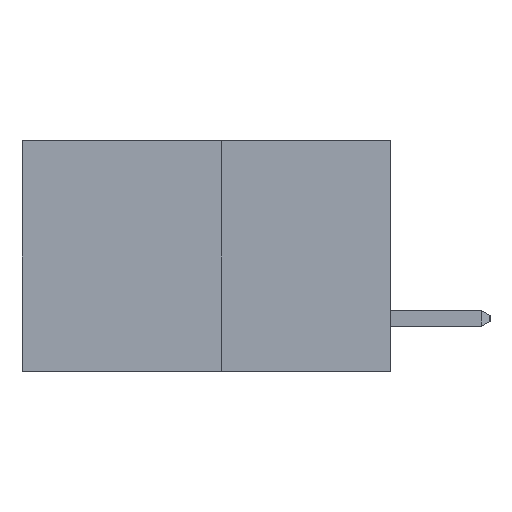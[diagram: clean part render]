
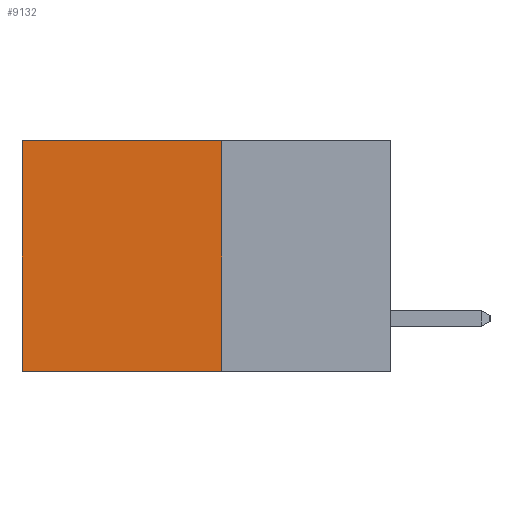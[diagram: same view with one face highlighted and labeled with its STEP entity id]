
A CAD part, left-side view. The second image highlights one B-rep face of the part: STEP entity #9132.
In plain terms, the highlighted planar face has unit normal (-1, 0, 0).
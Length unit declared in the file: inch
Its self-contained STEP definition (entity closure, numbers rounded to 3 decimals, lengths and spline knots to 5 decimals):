
#36 = EDGE_CURVE ( 'NONE', #1940, #594, #4179, .T. ) ;
#564 = EDGE_CURVE ( 'NONE', #12726, #3194, #19145, .T. ) ;
#594 = VERTEX_POINT ( 'NONE', #16345 ) ;
#688 = DIRECTION ( 'NONE',  ( 0., 0., -1. ) ) ;
#1038 = CARTESIAN_POINT ( 'NONE',  ( 0.277, 0.27, 0. ) ) ;
#1248 = DIRECTION ( 'NONE',  ( 1., 0., 0. ) ) ;
#1417 = DIRECTION ( 'NONE',  ( 0., 0., -1. ) ) ;
#1940 = VERTEX_POINT ( 'NONE', #5969 ) ;
#3194 = VERTEX_POINT ( 'NONE', #16776 ) ;
#3396 = EDGE_LOOP ( 'NONE', ( #16130, #18231, #19971, #7120 ) ) ;
#3668 = VECTOR ( 'NONE', #688, 39.37008 ) ;
#3925 = CARTESIAN_POINT ( 'NONE',  ( 0.277, 0.59, -0.37 ) ) ;
#4179 = LINE ( 'NONE', #3925, #3668 ) ;
#4764 = VECTOR ( 'NONE', #9232, 39.37008 ) ;
#5646 = CARTESIAN_POINT ( 'NONE',  ( 0.277, 0.27, -0.37 ) ) ;
#5954 = VECTOR ( 'NONE', #1417, 39.37008 ) ;
#5969 = CARTESIAN_POINT ( 'NONE',  ( 0.277, 0.59, 0. ) ) ;
#7120 = ORIENTED_EDGE ( 'NONE', *, *, #15231, .T. ) ;
#7750 = PLANE ( 'NONE',  #15616 ) ;
#9061 = LINE ( 'NONE', #15593, #4764 ) ;
#9132 = ADVANCED_FACE ( 'NONE', ( #12878 ), #7750, .F. ) ;
#9227 = CARTESIAN_POINT ( 'NONE',  ( 0.277, 0.27, 0. ) ) ;
#9232 = DIRECTION ( 'NONE',  ( 0., 1., 0. ) ) ;
#11045 = CARTESIAN_POINT ( 'NONE',  ( 0.277, 0.27, -0.37 ) ) ;
#12286 = VECTOR ( 'NONE', #20248, 39.37008 ) ;
#12632 = DIRECTION ( 'NONE',  ( 0., 0., -1. ) ) ;
#12726 = VERTEX_POINT ( 'NONE', #1038 ) ;
#12878 = FACE_OUTER_BOUND ( 'NONE', #3396, .T. ) ;
#15231 = EDGE_CURVE ( 'NONE', #12726, #1940, #19151, .T. ) ;
#15593 = CARTESIAN_POINT ( 'NONE',  ( 0.277, 0.27, -0.37 ) ) ;
#15616 = AXIS2_PLACEMENT_3D ( 'NONE', #11045, #1248, #12632 ) ;
#16130 = ORIENTED_EDGE ( 'NONE', *, *, #36, .T. ) ;
#16345 = CARTESIAN_POINT ( 'NONE',  ( 0.277, 0.59, -0.37 ) ) ;
#16776 = CARTESIAN_POINT ( 'NONE',  ( 0.277, 0.27, -0.37 ) ) ;
#17003 = EDGE_CURVE ( 'NONE', #3194, #594, #9061, .T. ) ;
#18231 = ORIENTED_EDGE ( 'NONE', *, *, #17003, .F. ) ;
#19145 = LINE ( 'NONE', #5646, #5954 ) ;
#19151 = LINE ( 'NONE', #9227, #12286 ) ;
#19971 = ORIENTED_EDGE ( 'NONE', *, *, #564, .F. ) ;
#20248 = DIRECTION ( 'NONE',  ( 0., 1., 0. ) ) ;
